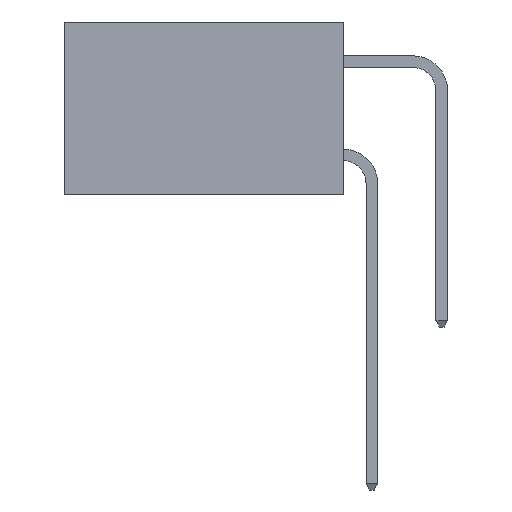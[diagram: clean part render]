
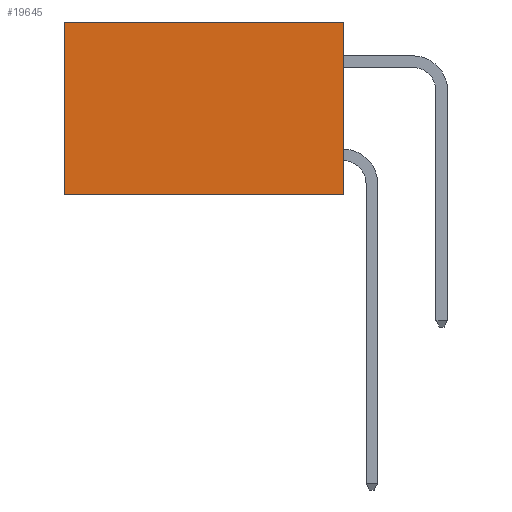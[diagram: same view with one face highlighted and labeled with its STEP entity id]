
A CAD part, left-side view. The second image highlights one B-rep face of the part: STEP entity #19645.
In plain terms, the highlighted planar face has unit normal (-1, 0, 0).
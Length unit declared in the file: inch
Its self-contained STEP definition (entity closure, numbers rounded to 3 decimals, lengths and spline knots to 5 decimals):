
#206 = CARTESIAN_POINT ( 'NONE',  ( 0.2615, 0., -0.37 ) ) ;
#1370 = VERTEX_POINT ( 'NONE', #22601 ) ;
#2434 = VECTOR ( 'NONE', #15511, 39.37008 ) ;
#2966 = AXIS2_PLACEMENT_3D ( 'NONE', #15382, #3150, #17364 ) ;
#3024 = LINE ( 'NONE', #13423, #2434 ) ;
#3150 = DIRECTION ( 'NONE',  ( 1., 0., 0. ) ) ;
#3745 = VERTEX_POINT ( 'NONE', #206 ) ;
#3949 = VERTEX_POINT ( 'NONE', #25774 ) ;
#4245 = VECTOR ( 'NONE', #23644, 39.37008 ) ;
#7541 = EDGE_CURVE ( 'NONE', #3949, #1370, #18277, .T. ) ;
#7574 = ORIENTED_EDGE ( 'NONE', *, *, #15022, .F. ) ;
#8971 = LINE ( 'NONE', #14150, #19594 ) ;
#11343 = PLANE ( 'NONE',  #2966 ) ;
#12135 = DIRECTION ( 'NONE',  ( 0., 0., -1. ) ) ;
#13423 = CARTESIAN_POINT ( 'NONE',  ( 0.2615, 0., -0.37 ) ) ;
#14150 = CARTESIAN_POINT ( 'NONE',  ( 0.2615, 0., -0.37 ) ) ;
#15022 = EDGE_CURVE ( 'NONE', #20128, #3745, #8971, .T. ) ;
#15382 = CARTESIAN_POINT ( 'NONE',  ( 0.2615, 0., -0.37 ) ) ;
#15511 = DIRECTION ( 'NONE',  ( 0., 1., 0. ) ) ;
#15551 = ORIENTED_EDGE ( 'NONE', *, *, #25083, .T. ) ;
#16656 = EDGE_LOOP ( 'NONE', ( #19777, #23085, #7574, #15551 ) ) ;
#17364 = DIRECTION ( 'NONE',  ( 0., 0., -1. ) ) ;
#18277 = LINE ( 'NONE', #23133, #19485 ) ;
#18661 = CARTESIAN_POINT ( 'NONE',  ( 0.2615, 0., 0. ) ) ;
#19485 = VECTOR ( 'NONE', #23161, 39.37008 ) ;
#19594 = VECTOR ( 'NONE', #12135, 39.37008 ) ;
#19645 = ADVANCED_FACE ( 'NONE', ( #24455 ), #11343, .F. ) ;
#19777 = ORIENTED_EDGE ( 'NONE', *, *, #7541, .T. ) ;
#20128 = VERTEX_POINT ( 'NONE', #18661 ) ;
#20353 = LINE ( 'NONE', #21672, #4245 ) ;
#21672 = CARTESIAN_POINT ( 'NONE',  ( 0.2615, 0., 0. ) ) ;
#22601 = CARTESIAN_POINT ( 'NONE',  ( 0.2615, 0.6, -0.37 ) ) ;
#23085 = ORIENTED_EDGE ( 'NONE', *, *, #23620, .F. ) ;
#23133 = CARTESIAN_POINT ( 'NONE',  ( 0.2615, 0.6, -0.37 ) ) ;
#23161 = DIRECTION ( 'NONE',  ( 0., 0., -1. ) ) ;
#23620 = EDGE_CURVE ( 'NONE', #3745, #1370, #3024, .T. ) ;
#23644 = DIRECTION ( 'NONE',  ( 0., 1., 0. ) ) ;
#24455 = FACE_OUTER_BOUND ( 'NONE', #16656, .T. ) ;
#25083 = EDGE_CURVE ( 'NONE', #20128, #3949, #20353, .T. ) ;
#25774 = CARTESIAN_POINT ( 'NONE',  ( 0.2615, 0.6, 0. ) ) ;
